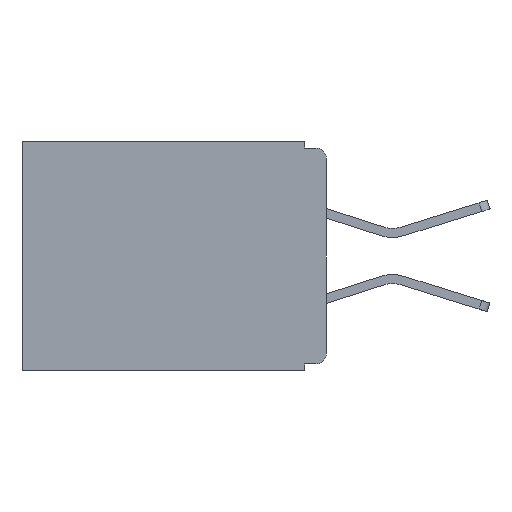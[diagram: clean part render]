
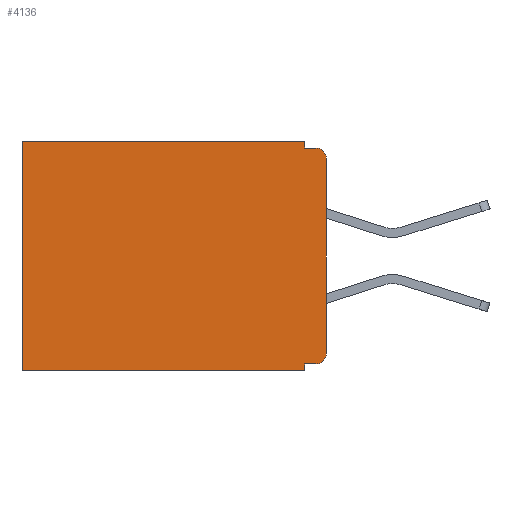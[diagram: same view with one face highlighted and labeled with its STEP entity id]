
A CAD part, left-side view. The second image highlights one B-rep face of the part: STEP entity #4136.
In plain terms, the highlighted planar face has unit normal (-1, 0, 0).
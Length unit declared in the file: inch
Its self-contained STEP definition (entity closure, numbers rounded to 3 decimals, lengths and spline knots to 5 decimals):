
#541 = VERTEX_POINT ( 'NONE', #3861 ) ;
#592 = EDGE_LOOP ( 'NONE', ( #12965, #24660, #23203, #21855, #5082, #17415, #2916, #5077, #19801, #22948 ) ) ;
#1499 = LINE ( 'NONE', #14844, #10604 ) ;
#1595 = DIRECTION ( 'NONE',  ( 0., 1., 0. ) ) ;
#1613 = EDGE_CURVE ( 'NONE', #16813, #13435, #1499, .T. ) ;
#1872 = CIRCLE ( 'NONE', #16802, 0.015 ) ;
#2639 = EDGE_CURVE ( 'NONE', #14380, #21669, #3568, .T. ) ;
#2732 = CARTESIAN_POINT ( 'NONE',  ( 0.3, 0., -0.025 ) ) ;
#2909 = VERTEX_POINT ( 'NONE', #2732 ) ;
#2916 = ORIENTED_EDGE ( 'NONE', *, *, #21173, .F. ) ;
#2984 = VECTOR ( 'NONE', #7563, 39.37008 ) ;
#3302 = CARTESIAN_POINT ( 'NONE',  ( 0.3, 0.015, -0.32 ) ) ;
#3568 = LINE ( 'NONE', #19903, #2984 ) ;
#3861 = CARTESIAN_POINT ( 'NONE',  ( 0.3, 0.015, -0.01 ) ) ;
#3976 = AXIS2_PLACEMENT_3D ( 'NONE', #12396, #17916, #17888 ) ;
#4019 = EDGE_CURVE ( 'NONE', #16813, #23820, #8045, .T. ) ;
#4136 = ADVANCED_FACE ( 'NONE', ( #15280 ), #24840, .F. ) ;
#4474 = VERTEX_POINT ( 'NONE', #3302 ) ;
#5024 = CARTESIAN_POINT ( 'NONE',  ( 0.3, 0.015, -0.305 ) ) ;
#5077 = ORIENTED_EDGE ( 'NONE', *, *, #2639, .F. ) ;
#5082 = ORIENTED_EDGE ( 'NONE', *, *, #4019, .T. ) ;
#5238 = CARTESIAN_POINT ( 'NONE',  ( 0.3, 0.437, -0.33 ) ) ;
#5303 = VECTOR ( 'NONE', #1595, 39.37008 ) ;
#6000 = CARTESIAN_POINT ( 'NONE',  ( 0.3, 0.031, -0.32 ) ) ;
#6334 = CARTESIAN_POINT ( 'NONE',  ( 0.3, 0.437, -0.33 ) ) ;
#6555 = VECTOR ( 'NONE', #18682, 39.37008 ) ;
#6718 = DIRECTION ( 'NONE',  ( 0., 1., 0. ) ) ;
#6737 = CARTESIAN_POINT ( 'NONE',  ( 0.3, 0., 0. ) ) ;
#7012 = DIRECTION ( 'NONE',  ( 0., 0., -1. ) ) ;
#7563 = DIRECTION ( 'NONE',  ( 0., 0., -1. ) ) ;
#8045 = LINE ( 'NONE', #6737, #13209 ) ;
#8187 = DIRECTION ( 'NONE',  ( 0., 0., -1. ) ) ;
#8292 = DIRECTION ( 'NONE',  ( 0., 0., -1. ) ) ;
#8762 = EDGE_CURVE ( 'NONE', #2909, #541, #21929, .T. ) ;
#9016 = CARTESIAN_POINT ( 'NONE',  ( 0.3, 0.031, -0.33 ) ) ;
#10123 = DIRECTION ( 'NONE',  ( 0., 0., -1. ) ) ;
#10604 = VECTOR ( 'NONE', #10123, 39.37008 ) ;
#10981 = VERTEX_POINT ( 'NONE', #5238 ) ;
#11170 = VECTOR ( 'NONE', #8292, 39.37008 ) ;
#11365 = EDGE_CURVE ( 'NONE', #4474, #14380, #11699, .T. ) ;
#11699 = LINE ( 'NONE', #19167, #6555 ) ;
#12396 = CARTESIAN_POINT ( 'NONE',  ( 0.3, 0., -0.33 ) ) ;
#12609 = DIRECTION ( 'NONE',  ( 0., -1., 0. ) ) ;
#12647 = CARTESIAN_POINT ( 'NONE',  ( 0.3, 0.015, -0.025 ) ) ;
#12742 = EDGE_CURVE ( 'NONE', #13435, #541, #20301, .T. ) ;
#12965 = ORIENTED_EDGE ( 'NONE', *, *, #13250, .F. ) ;
#13209 = VECTOR ( 'NONE', #6718, 39.37008 ) ;
#13250 = EDGE_CURVE ( 'NONE', #2909, #22837, #19688, .T. ) ;
#13435 = VERTEX_POINT ( 'NONE', #20471 ) ;
#14380 = VERTEX_POINT ( 'NONE', #6000 ) ;
#14649 = EDGE_CURVE ( 'NONE', #4474, #22837, #1872, .T. ) ;
#14844 = CARTESIAN_POINT ( 'NONE',  ( 0.3, 0.031, 0. ) ) ;
#14975 = CARTESIAN_POINT ( 'NONE',  ( 0.3, 0., -0.305 ) ) ;
#15280 = FACE_OUTER_BOUND ( 'NONE', #592, .T. ) ;
#16080 = AXIS2_PLACEMENT_3D ( 'NONE', #12647, #17399, #21316 ) ;
#16220 = LINE ( 'NONE', #18934, #5303 ) ;
#16802 = AXIS2_PLACEMENT_3D ( 'NONE', #5024, #18530, #7012 ) ;
#16813 = VERTEX_POINT ( 'NONE', #19511 ) ;
#16863 = LINE ( 'NONE', #6334, #11170 ) ;
#17399 = DIRECTION ( 'NONE',  ( -1., 0., 0. ) ) ;
#17415 = ORIENTED_EDGE ( 'NONE', *, *, #20277, .T. ) ;
#17888 = DIRECTION ( 'NONE',  ( 0., 0., -1. ) ) ;
#17916 = DIRECTION ( 'NONE',  ( 1., 0., 0. ) ) ;
#18530 = DIRECTION ( 'NONE',  ( -1., 0., 0. ) ) ;
#18682 = DIRECTION ( 'NONE',  ( 0., 1., 0. ) ) ;
#18934 = CARTESIAN_POINT ( 'NONE',  ( 0.3, 0., -0.33 ) ) ;
#19167 = CARTESIAN_POINT ( 'NONE',  ( 0.3, 0., -0.32 ) ) ;
#19511 = CARTESIAN_POINT ( 'NONE',  ( 0.3, 0.031, 0. ) ) ;
#19688 = LINE ( 'NONE', #23436, #24085 ) ;
#19801 = ORIENTED_EDGE ( 'NONE', *, *, #11365, .F. ) ;
#19903 = CARTESIAN_POINT ( 'NONE',  ( 0.3, 0.031, -0.33 ) ) ;
#20277 = EDGE_CURVE ( 'NONE', #23820, #10981, #16863, .T. ) ;
#20301 = LINE ( 'NONE', #23936, #21477 ) ;
#20471 = CARTESIAN_POINT ( 'NONE',  ( 0.3, 0.031, -0.01 ) ) ;
#21173 = EDGE_CURVE ( 'NONE', #21669, #10981, #16220, .T. ) ;
#21316 = DIRECTION ( 'NONE',  ( 0., 0., -1. ) ) ;
#21477 = VECTOR ( 'NONE', #12609, 39.37008 ) ;
#21608 = CARTESIAN_POINT ( 'NONE',  ( 0.3, 0.437, 0. ) ) ;
#21669 = VERTEX_POINT ( 'NONE', #9016 ) ;
#21855 = ORIENTED_EDGE ( 'NONE', *, *, #1613, .F. ) ;
#21929 = CIRCLE ( 'NONE', #16080, 0.015 ) ;
#22837 = VERTEX_POINT ( 'NONE', #14975 ) ;
#22948 = ORIENTED_EDGE ( 'NONE', *, *, #14649, .T. ) ;
#23203 = ORIENTED_EDGE ( 'NONE', *, *, #12742, .F. ) ;
#23436 = CARTESIAN_POINT ( 'NONE',  ( 0.3, 0., -0.33 ) ) ;
#23820 = VERTEX_POINT ( 'NONE', #21608 ) ;
#23936 = CARTESIAN_POINT ( 'NONE',  ( 0.3, 0., -0.01 ) ) ;
#24085 = VECTOR ( 'NONE', #8187, 39.37008 ) ;
#24660 = ORIENTED_EDGE ( 'NONE', *, *, #8762, .T. ) ;
#24840 = PLANE ( 'NONE',  #3976 ) ;
